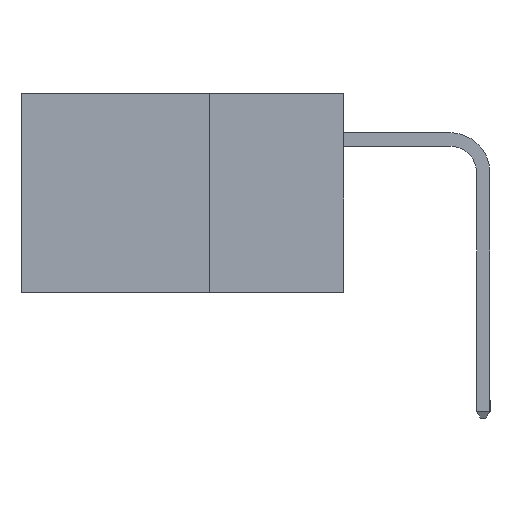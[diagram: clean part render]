
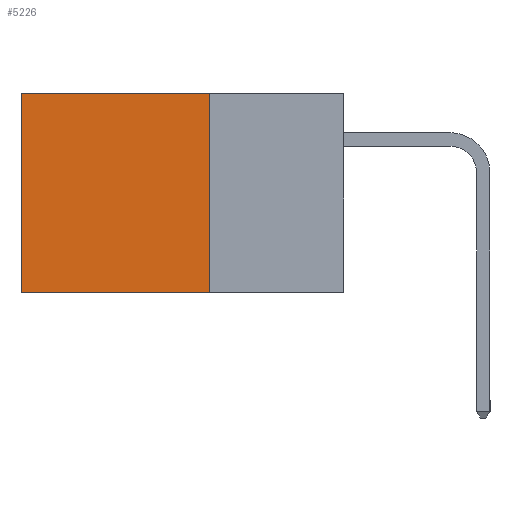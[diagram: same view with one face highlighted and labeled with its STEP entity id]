
A CAD part, left-side view. The second image highlights one B-rep face of the part: STEP entity #5226.
In plain terms, the highlighted planar face has unit normal (-1, 0, 0).
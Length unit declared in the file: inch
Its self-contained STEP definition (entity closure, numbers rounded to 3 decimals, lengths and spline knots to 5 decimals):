
#305 = VECTOR ( 'NONE', #6132, 39.37008 ) ;
#321 = VERTEX_POINT ( 'NONE', #11360 ) ;
#986 = CARTESIAN_POINT ( 'NONE',  ( 0.2615, 0.25, -0.37 ) ) ;
#1080 = DIRECTION ( 'NONE',  ( 0., 0., -1. ) ) ;
#1506 = VERTEX_POINT ( 'NONE', #10642 ) ;
#1775 = LINE ( 'NONE', #3224, #9252 ) ;
#1893 = ORIENTED_EDGE ( 'NONE', *, *, #4404, .F. ) ;
#2109 = EDGE_CURVE ( 'NONE', #321, #3055, #3854, .T. ) ;
#2715 = EDGE_CURVE ( 'NONE', #1506, #321, #5556, .T. ) ;
#3038 = VECTOR ( 'NONE', #1080, 39.37008 ) ;
#3055 = VERTEX_POINT ( 'NONE', #12369 ) ;
#3224 = CARTESIAN_POINT ( 'NONE',  ( 0.2615, 0.25, -0.37 ) ) ;
#3571 = CARTESIAN_POINT ( 'NONE',  ( 0.2615, 0.25, -0.37 ) ) ;
#3637 = LINE ( 'NONE', #986, #3038 ) ;
#3854 = LINE ( 'NONE', #7470, #9029 ) ;
#4224 = ORIENTED_EDGE ( 'NONE', *, *, #2109, .T. ) ;
#4250 = EDGE_CURVE ( 'NONE', #1506, #11753, #3637, .T. ) ;
#4399 = FACE_OUTER_BOUND ( 'NONE', #5528, .T. ) ;
#4404 = EDGE_CURVE ( 'NONE', #11753, #3055, #1775, .T. ) ;
#4587 = DIRECTION ( 'NONE',  ( 0., 0., -1. ) ) ;
#5226 = ADVANCED_FACE ( 'NONE', ( #4399 ), #5546, .F. ) ;
#5528 = EDGE_LOOP ( 'NONE', ( #4224, #1893, #8060, #5645 ) ) ;
#5546 = PLANE ( 'NONE',  #8773 ) ;
#5556 = LINE ( 'NONE', #6221, #305 ) ;
#5645 = ORIENTED_EDGE ( 'NONE', *, *, #2715, .T. ) ;
#6132 = DIRECTION ( 'NONE',  ( 0., 1., 0. ) ) ;
#6221 = CARTESIAN_POINT ( 'NONE',  ( 0.2615, 0.25, 0. ) ) ;
#6836 = DIRECTION ( 'NONE',  ( 0., 0., -1. ) ) ;
#7470 = CARTESIAN_POINT ( 'NONE',  ( 0.2615, 0.6, -0.37 ) ) ;
#8060 = ORIENTED_EDGE ( 'NONE', *, *, #4250, .F. ) ;
#8773 = AXIS2_PLACEMENT_3D ( 'NONE', #3571, #10335, #4587 ) ;
#9029 = VECTOR ( 'NONE', #6836, 39.37008 ) ;
#9252 = VECTOR ( 'NONE', #9984, 39.37008 ) ;
#9871 = CARTESIAN_POINT ( 'NONE',  ( 0.2615, 0.25, -0.37 ) ) ;
#9984 = DIRECTION ( 'NONE',  ( 0., 1., 0. ) ) ;
#10335 = DIRECTION ( 'NONE',  ( 1., 0., 0. ) ) ;
#10642 = CARTESIAN_POINT ( 'NONE',  ( 0.2615, 0.25, 0. ) ) ;
#11360 = CARTESIAN_POINT ( 'NONE',  ( 0.2615, 0.6, 0. ) ) ;
#11753 = VERTEX_POINT ( 'NONE', #9871 ) ;
#12369 = CARTESIAN_POINT ( 'NONE',  ( 0.2615, 0.6, -0.37 ) ) ;
